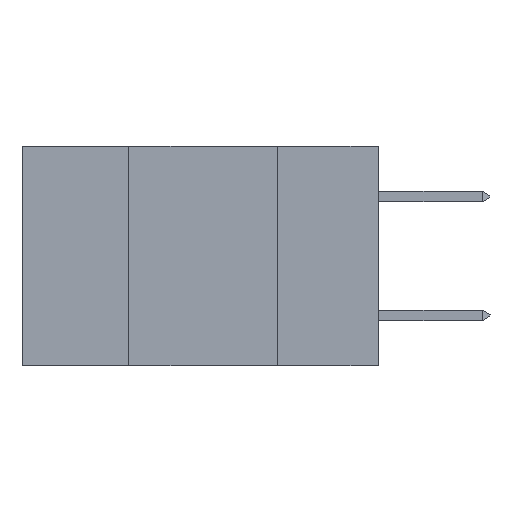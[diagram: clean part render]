
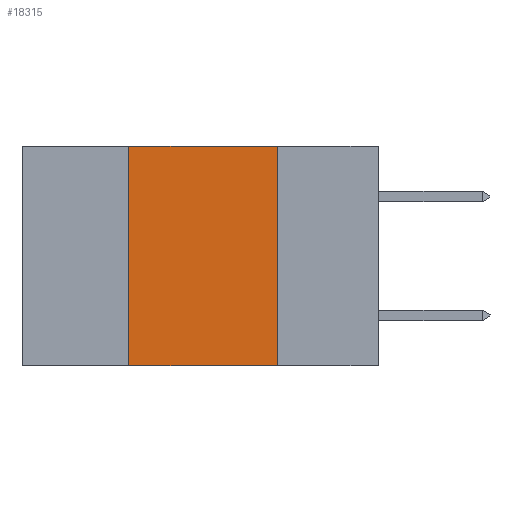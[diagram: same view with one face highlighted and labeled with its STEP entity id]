
A CAD part, left-side view. The second image highlights one B-rep face of the part: STEP entity #18315.
In plain terms, the highlighted planar face has unit normal (-1, 0, 0).
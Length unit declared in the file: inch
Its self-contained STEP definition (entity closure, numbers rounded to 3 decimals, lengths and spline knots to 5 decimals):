
#202 = VECTOR ( 'NONE', #17736, 39.37008 ) ;
#740 = DIRECTION ( 'NONE',  ( 0., 0., -1. ) ) ;
#1897 = DIRECTION ( 'NONE',  ( 0., 0., -1. ) ) ;
#4563 = CARTESIAN_POINT ( 'NONE',  ( 0., 0.17, 0. ) ) ;
#6605 = AXIS2_PLACEMENT_3D ( 'NONE', #9894, #33737, #1897 ) ;
#6642 = CARTESIAN_POINT ( 'NONE',  ( 0., 0.6, 0. ) ) ;
#7421 = VERTEX_POINT ( 'NONE', #10252 ) ;
#7655 = VECTOR ( 'NONE', #33874, 39.37008 ) ;
#8773 = CARTESIAN_POINT ( 'NONE',  ( 0., 0.42, 0. ) ) ;
#8928 = VECTOR ( 'NONE', #740, 39.37008 ) ;
#9894 = CARTESIAN_POINT ( 'NONE',  ( 0., 0.6, 0. ) ) ;
#10172 = LINE ( 'NONE', #17832, #7655 ) ;
#10252 = CARTESIAN_POINT ( 'NONE',  ( 0., 0.42, -0.37 ) ) ;
#10943 = EDGE_CURVE ( 'NONE', #27658, #31976, #27434, .T. ) ;
#11529 = LINE ( 'NONE', #6642, #202 ) ;
#11694 = VERTEX_POINT ( 'NONE', #12411 ) ;
#11786 = EDGE_LOOP ( 'NONE', ( #25986, #15410, #15054, #17107 ) ) ;
#12411 = CARTESIAN_POINT ( 'NONE',  ( 0., 0.42, 0. ) ) ;
#14102 = DIRECTION ( 'NONE',  ( 0., 0., 1. ) ) ;
#14397 = LINE ( 'NONE', #8773, #30272 ) ;
#15054 = ORIENTED_EDGE ( 'NONE', *, *, #28077, .F. ) ;
#15410 = ORIENTED_EDGE ( 'NONE', *, *, #26787, .F. ) ;
#17107 = ORIENTED_EDGE ( 'NONE', *, *, #30695, .T. ) ;
#17736 = DIRECTION ( 'NONE',  ( 0., -1., 0. ) ) ;
#17832 = CARTESIAN_POINT ( 'NONE',  ( 0., 0.6, -0.37 ) ) ;
#17865 = CARTESIAN_POINT ( 'NONE',  ( 0., 0.17, -0.37 ) ) ;
#18315 = ADVANCED_FACE ( 'NONE', ( #32321 ), #33613, .F. ) ;
#25986 = ORIENTED_EDGE ( 'NONE', *, *, #10943, .F. ) ;
#26787 = EDGE_CURVE ( 'NONE', #11694, #27658, #11529, .T. ) ;
#27434 = LINE ( 'NONE', #32708, #8928 ) ;
#27658 = VERTEX_POINT ( 'NONE', #4563 ) ;
#28077 = EDGE_CURVE ( 'NONE', #7421, #11694, #14397, .T. ) ;
#30272 = VECTOR ( 'NONE', #14102, 39.37008 ) ;
#30695 = EDGE_CURVE ( 'NONE', #7421, #31976, #10172, .T. ) ;
#31976 = VERTEX_POINT ( 'NONE', #17865 ) ;
#32321 = FACE_OUTER_BOUND ( 'NONE', #11786, .T. ) ;
#32708 = CARTESIAN_POINT ( 'NONE',  ( 0., 0.17, 0. ) ) ;
#33613 = PLANE ( 'NONE',  #6605 ) ;
#33737 = DIRECTION ( 'NONE',  ( 1., 0., 0. ) ) ;
#33874 = DIRECTION ( 'NONE',  ( 0., -1., 0. ) ) ;
